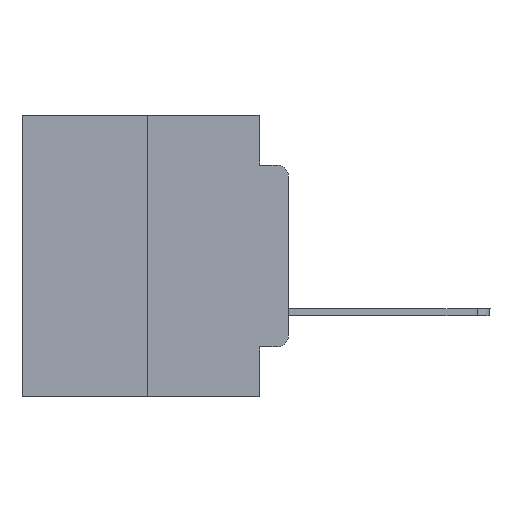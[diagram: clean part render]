
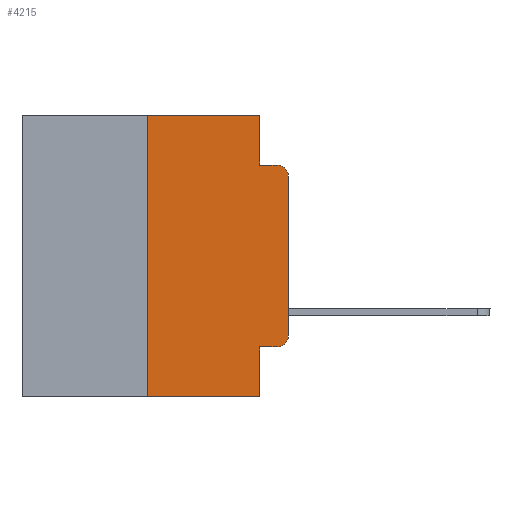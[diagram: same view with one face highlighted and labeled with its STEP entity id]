
A CAD part, left-side view. The second image highlights one B-rep face of the part: STEP entity #4215.
In plain terms, the highlighted planar face has unit normal (-1, 0, 0).
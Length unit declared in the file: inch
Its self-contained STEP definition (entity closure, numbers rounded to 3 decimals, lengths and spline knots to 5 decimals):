
#162 = CARTESIAN_POINT ( 'NONE',  ( 0., 0.02, -0.3915 ) ) ;
#569 = CARTESIAN_POINT ( 'NONE',  ( 0., 0.473, -0.5 ) ) ;
#797 = VECTOR ( 'NONE', #12285, 39.37008 ) ;
#2271 = VERTEX_POINT ( 'NONE', #13548 ) ;
#2371 = ORIENTED_EDGE ( 'NONE', *, *, #14676, .T. ) ;
#2481 = VERTEX_POINT ( 'NONE', #8532 ) ;
#2701 = EDGE_CURVE ( 'NONE', #2271, #8292, #26972, .T. ) ;
#3011 = LINE ( 'NONE', #22412, #9867 ) ;
#3043 = DIRECTION ( 'NONE',  ( 0., 0., -1. ) ) ;
#3494 = VECTOR ( 'NONE', #23960, 39.37008 ) ;
#3624 = ORIENTED_EDGE ( 'NONE', *, *, #7101, .T. ) ;
#4061 = VERTEX_POINT ( 'NONE', #11906 ) ;
#4215 = ADVANCED_FACE ( 'NONE', ( #14839 ), #25866, .F. ) ;
#4508 = DIRECTION ( 'NONE',  ( -1., 0., 0. ) ) ;
#4612 = CARTESIAN_POINT ( 'NONE',  ( 0., 0., -0.1085 ) ) ;
#4769 = CARTESIAN_POINT ( 'NONE',  ( 0., 0.473, 0. ) ) ;
#4810 = DIRECTION ( 'NONE',  ( 0., -1., 0. ) ) ;
#4962 = LINE ( 'NONE', #13475, #3494 ) ;
#5231 = CARTESIAN_POINT ( 'NONE',  ( 0., 0.25, -0.5 ) ) ;
#5882 = EDGE_CURVE ( 'NONE', #12666, #2481, #8533, .T. ) ;
#5941 = VECTOR ( 'NONE', #8863, 39.37008 ) ;
#6478 = ORIENTED_EDGE ( 'NONE', *, *, #2701, .F. ) ;
#6906 = EDGE_LOOP ( 'NONE', ( #7269, #3624, #22108, #6478, #26487, #26387, #21125, #8715, #27431, #2371 ) ) ;
#7101 = EDGE_CURVE ( 'NONE', #23367, #4061, #8708, .T. ) ;
#7226 = CARTESIAN_POINT ( 'NONE',  ( 0., 0.02, -0.1085 ) ) ;
#7269 = ORIENTED_EDGE ( 'NONE', *, *, #13740, .T. ) ;
#7990 = AXIS2_PLACEMENT_3D ( 'NONE', #4769, #26402, #9241 ) ;
#8292 = VERTEX_POINT ( 'NONE', #14658 ) ;
#8532 = CARTESIAN_POINT ( 'NONE',  ( 0., 0.25, 0. ) ) ;
#8533 = LINE ( 'NONE', #25688, #797 ) ;
#8708 = CIRCLE ( 'NONE', #11816, 0.02 ) ;
#8715 = ORIENTED_EDGE ( 'NONE', *, *, #22402, .F. ) ;
#8863 = DIRECTION ( 'NONE',  ( 0., -1., 0. ) ) ;
#9241 = DIRECTION ( 'NONE',  ( 0., 0., -1. ) ) ;
#9867 = VECTOR ( 'NONE', #26454, 39.37008 ) ;
#10888 = CARTESIAN_POINT ( 'NONE',  ( 0., 0., 0. ) ) ;
#11035 = VECTOR ( 'NONE', #25544, 39.37008 ) ;
#11225 = CARTESIAN_POINT ( 'NONE',  ( 0., 0.051, -0.4115 ) ) ;
#11276 = EDGE_CURVE ( 'NONE', #8292, #4061, #4962, .T. ) ;
#11816 = AXIS2_PLACEMENT_3D ( 'NONE', #7226, #24262, #3043 ) ;
#11906 = CARTESIAN_POINT ( 'NONE',  ( 0., 0.02, -0.0885 ) ) ;
#11959 = VECTOR ( 'NONE', #4810, 39.37008 ) ;
#12157 = VERTEX_POINT ( 'NONE', #15248 ) ;
#12285 = DIRECTION ( 'NONE',  ( 0., 0., 1. ) ) ;
#12550 = VECTOR ( 'NONE', #17914, 39.37008 ) ;
#12666 = VERTEX_POINT ( 'NONE', #5231 ) ;
#13414 = EDGE_CURVE ( 'NONE', #12666, #20695, #19723, .T. ) ;
#13475 = CARTESIAN_POINT ( 'NONE',  ( 0., 0.051, -0.0885 ) ) ;
#13548 = CARTESIAN_POINT ( 'NONE',  ( 0., 0.051, 0. ) ) ;
#13740 = EDGE_CURVE ( 'NONE', #21605, #23367, #21381, .T. ) ;
#13858 = CARTESIAN_POINT ( 'NONE',  ( 0., 0., -0.3915 ) ) ;
#13924 = CARTESIAN_POINT ( 'NONE',  ( 0., 0.051, -0.5 ) ) ;
#14658 = CARTESIAN_POINT ( 'NONE',  ( 0., 0.051, -0.0885 ) ) ;
#14676 = EDGE_CURVE ( 'NONE', #12157, #21605, #27589, .T. ) ;
#14839 = FACE_OUTER_BOUND ( 'NONE', #6906, .T. ) ;
#15248 = CARTESIAN_POINT ( 'NONE',  ( 0., 0.02, -0.4115 ) ) ;
#15793 = DIRECTION ( 'NONE',  ( 0., 0., -1. ) ) ;
#15819 = CARTESIAN_POINT ( 'NONE',  ( 0., 0.051, 0. ) ) ;
#16114 = EDGE_CURVE ( 'NONE', #2481, #2271, #17519, .T. ) ;
#17254 = VECTOR ( 'NONE', #25716, 39.37008 ) ;
#17270 = CARTESIAN_POINT ( 'NONE',  ( 0., 0.051, -0.4115 ) ) ;
#17519 = LINE ( 'NONE', #26310, #11959 ) ;
#17630 = LINE ( 'NONE', #11225, #5941 ) ;
#17914 = DIRECTION ( 'NONE',  ( 0., 0., -1. ) ) ;
#19107 = AXIS2_PLACEMENT_3D ( 'NONE', #162, #4508, #15793 ) ;
#19723 = LINE ( 'NONE', #569, #17254 ) ;
#20695 = VERTEX_POINT ( 'NONE', #13924 ) ;
#21125 = ORIENTED_EDGE ( 'NONE', *, *, #13414, .T. ) ;
#21381 = LINE ( 'NONE', #10888, #11035 ) ;
#21605 = VERTEX_POINT ( 'NONE', #13858 ) ;
#22108 = ORIENTED_EDGE ( 'NONE', *, *, #11276, .F. ) ;
#22291 = VERTEX_POINT ( 'NONE', #17270 ) ;
#22402 = EDGE_CURVE ( 'NONE', #22291, #20695, #3011, .T. ) ;
#22412 = CARTESIAN_POINT ( 'NONE',  ( 0., 0.051, 0. ) ) ;
#23367 = VERTEX_POINT ( 'NONE', #4612 ) ;
#23960 = DIRECTION ( 'NONE',  ( 0., -1., 0. ) ) ;
#24262 = DIRECTION ( 'NONE',  ( -1., 0., 0. ) ) ;
#25544 = DIRECTION ( 'NONE',  ( 0., 0., 1. ) ) ;
#25688 = CARTESIAN_POINT ( 'NONE',  ( 0., 0.25, 0. ) ) ;
#25716 = DIRECTION ( 'NONE',  ( 0., -1., 0. ) ) ;
#25866 = PLANE ( 'NONE',  #7990 ) ;
#25972 = EDGE_CURVE ( 'NONE', #22291, #12157, #17630, .T. ) ;
#26310 = CARTESIAN_POINT ( 'NONE',  ( 0., 0.473, 0. ) ) ;
#26387 = ORIENTED_EDGE ( 'NONE', *, *, #5882, .F. ) ;
#26402 = DIRECTION ( 'NONE',  ( 1., 0., 0. ) ) ;
#26454 = DIRECTION ( 'NONE',  ( 0., 0., -1. ) ) ;
#26487 = ORIENTED_EDGE ( 'NONE', *, *, #16114, .F. ) ;
#26972 = LINE ( 'NONE', #15819, #12550 ) ;
#27431 = ORIENTED_EDGE ( 'NONE', *, *, #25972, .T. ) ;
#27589 = CIRCLE ( 'NONE', #19107, 0.02 ) ;
